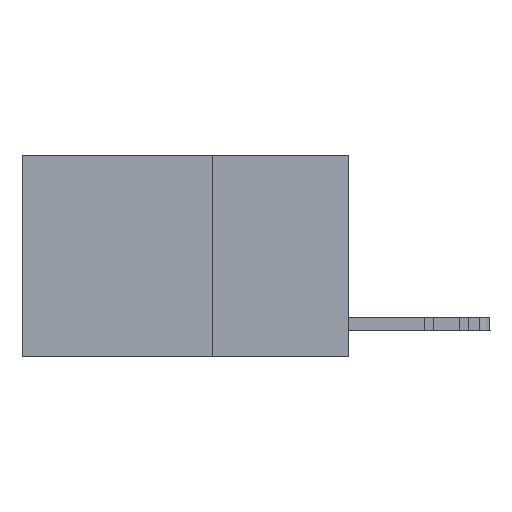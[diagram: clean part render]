
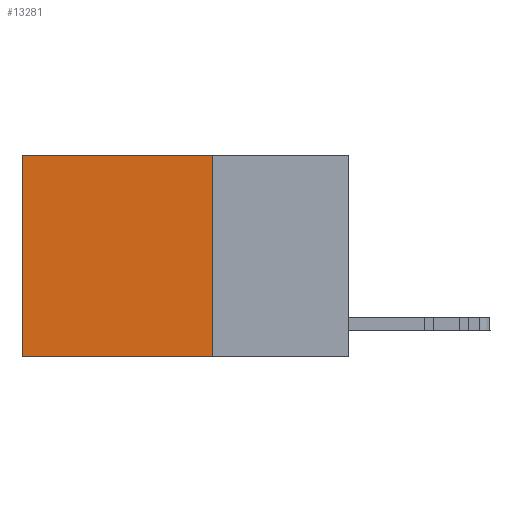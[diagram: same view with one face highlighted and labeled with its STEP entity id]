
A CAD part, left-side view. The second image highlights one B-rep face of the part: STEP entity #13281.
In plain terms, the highlighted planar face has unit normal (-1, 0, 0).
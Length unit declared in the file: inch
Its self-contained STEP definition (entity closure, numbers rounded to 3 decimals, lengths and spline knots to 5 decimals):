
#659 = DIRECTION ( 'NONE',  ( 0., 0., -1. ) ) ;
#1244 = DIRECTION ( 'NONE',  ( 0., 0., -1. ) ) ;
#1713 = ORIENTED_EDGE ( 'NONE', *, *, #16796, .F. ) ;
#2270 = CARTESIAN_POINT ( 'NONE',  ( 0.2625, 0.6, -0.37 ) ) ;
#3177 = CARTESIAN_POINT ( 'NONE',  ( 0.2625, 0.25, 0. ) ) ;
#3280 = CARTESIAN_POINT ( 'NONE',  ( 0.2625, 0.6, 0. ) ) ;
#3364 = LINE ( 'NONE', #8193, #20808 ) ;
#4807 = EDGE_LOOP ( 'NONE', ( #8713, #22403, #1713, #26784 ) ) ;
#4855 = VERTEX_POINT ( 'NONE', #3280 ) ;
#4991 = EDGE_CURVE ( 'NONE', #4855, #5499, #15054, .T. ) ;
#5194 = EDGE_CURVE ( 'NONE', #20515, #5499, #3364, .T. ) ;
#5499 = VERTEX_POINT ( 'NONE', #2270 ) ;
#5826 = EDGE_CURVE ( 'NONE', #7997, #4855, #21362, .T. ) ;
#6076 = DIRECTION ( 'NONE',  ( 0., 1., 0. ) ) ;
#6366 = CARTESIAN_POINT ( 'NONE',  ( 0.2625, 0.25, 0. ) ) ;
#7316 = FACE_OUTER_BOUND ( 'NONE', #4807, .T. ) ;
#7997 = VERTEX_POINT ( 'NONE', #23582 ) ;
#8193 = CARTESIAN_POINT ( 'NONE',  ( 0.2625, 0.25, -0.37 ) ) ;
#8713 = ORIENTED_EDGE ( 'NONE', *, *, #4991, .T. ) ;
#10370 = AXIS2_PLACEMENT_3D ( 'NONE', #3177, #11278, #659 ) ;
#11278 = DIRECTION ( 'NONE',  ( 1., 0., 0. ) ) ;
#11743 = VECTOR ( 'NONE', #15179, 39.37008 ) ;
#12295 = LINE ( 'NONE', #20779, #15867 ) ;
#13281 = ADVANCED_FACE ( 'NONE', ( #7316 ), #13824, .F. ) ;
#13824 = PLANE ( 'NONE',  #10370 ) ;
#15054 = LINE ( 'NONE', #21120, #11743 ) ;
#15165 = VECTOR ( 'NONE', #25478, 39.37008 ) ;
#15179 = DIRECTION ( 'NONE',  ( 0., 0., -1. ) ) ;
#15790 = CARTESIAN_POINT ( 'NONE',  ( 0.2625, 0.25, -0.37 ) ) ;
#15867 = VECTOR ( 'NONE', #1244, 39.37008 ) ;
#16796 = EDGE_CURVE ( 'NONE', #7997, #20515, #12295, .T. ) ;
#20515 = VERTEX_POINT ( 'NONE', #15790 ) ;
#20779 = CARTESIAN_POINT ( 'NONE',  ( 0.2625, 0.25, 0. ) ) ;
#20808 = VECTOR ( 'NONE', #6076, 39.37008 ) ;
#21120 = CARTESIAN_POINT ( 'NONE',  ( 0.2625, 0.6, 0. ) ) ;
#21362 = LINE ( 'NONE', #6366, #15165 ) ;
#22403 = ORIENTED_EDGE ( 'NONE', *, *, #5194, .F. ) ;
#23582 = CARTESIAN_POINT ( 'NONE',  ( 0.2625, 0.25, 0. ) ) ;
#25478 = DIRECTION ( 'NONE',  ( 0., 1., 0. ) ) ;
#26784 = ORIENTED_EDGE ( 'NONE', *, *, #5826, .T. ) ;
